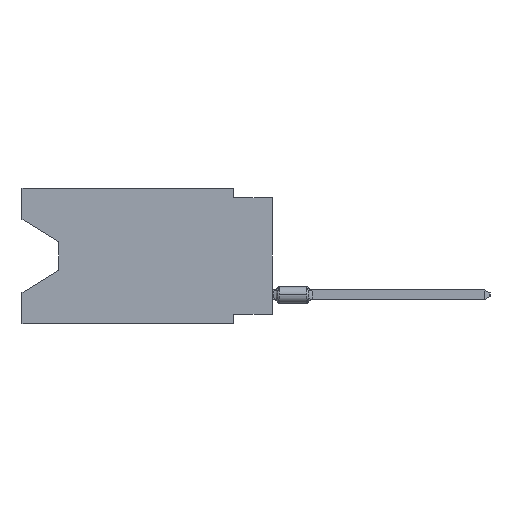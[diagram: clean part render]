
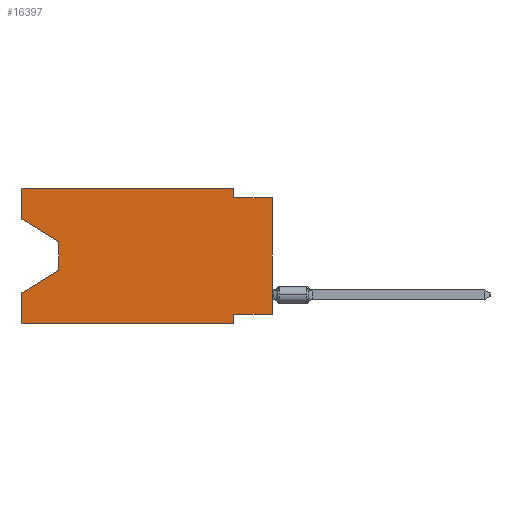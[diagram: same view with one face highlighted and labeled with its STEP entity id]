
A CAD part, left-side view. The second image highlights one B-rep face of the part: STEP entity #16397.
In plain terms, the highlighted planar face has unit normal (-1, 0, 0).
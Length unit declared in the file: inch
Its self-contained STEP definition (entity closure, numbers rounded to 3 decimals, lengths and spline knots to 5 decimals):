
#1196 = DIRECTION ( 'NONE',  ( 0., 0., -1. ) ) ;
#1961 = EDGE_CURVE ( 'NONE', #27140, #8039, #2469, .T. ) ;
#2184 = VECTOR ( 'NONE', #6660, 39.37008 ) ;
#2469 = LINE ( 'NONE', #33459, #2823 ) ;
#2578 = DIRECTION ( 'NONE',  ( 0., 1., 0. ) ) ;
#2591 = CARTESIAN_POINT ( 'NONE',  ( 0., 0., -0.025 ) ) ;
#2623 = VECTOR ( 'NONE', #19861, 39.37008 ) ;
#2651 = ORIENTED_EDGE ( 'NONE', *, *, #20667, .T. ) ;
#2823 = VECTOR ( 'NONE', #5797, 39.37008 ) ;
#2861 = CARTESIAN_POINT ( 'NONE',  ( 0., 0.645, -0.35 ) ) ;
#3472 = CARTESIAN_POINT ( 'NONE',  ( 0., 0.55, -0.138 ) ) ;
#3521 = FACE_OUTER_BOUND ( 'NONE', #13772, .T. ) ;
#3832 = VERTEX_POINT ( 'NONE', #13903 ) ;
#3996 = ORIENTED_EDGE ( 'NONE', *, *, #23947, .F. ) ;
#4354 = VECTOR ( 'NONE', #19300, 39.37008 ) ;
#4499 = ORIENTED_EDGE ( 'NONE', *, *, #34198, .F. ) ;
#4878 = CARTESIAN_POINT ( 'NONE',  ( 0., 0.1, -0.325 ) ) ;
#5626 = ORIENTED_EDGE ( 'NONE', *, *, #24805, .T. ) ;
#5797 = DIRECTION ( 'NONE',  ( 0., 0., -1. ) ) ;
#5922 = CARTESIAN_POINT ( 'NONE',  ( 0., 0., 0. ) ) ;
#6173 = VERTEX_POINT ( 'NONE', #33306 ) ;
#6267 = VECTOR ( 'NONE', #35871, 39.37008 ) ;
#6556 = LINE ( 'NONE', #35153, #23487 ) ;
#6660 = DIRECTION ( 'NONE',  ( 0., 0., 1. ) ) ;
#6826 = EDGE_CURVE ( 'NONE', #9993, #15553, #34733, .T. ) ;
#7477 = LINE ( 'NONE', #18599, #6267 ) ;
#7908 = VECTOR ( 'NONE', #35637, 39.37008 ) ;
#8039 = VERTEX_POINT ( 'NONE', #25841 ) ;
#8499 = VECTOR ( 'NONE', #20613, 39.37008 ) ;
#9249 = VECTOR ( 'NONE', #2578, 39.37008 ) ;
#9289 = CARTESIAN_POINT ( 'NONE',  ( 0., 0.645, -0.08025 ) ) ;
#9309 = CARTESIAN_POINT ( 'NONE',  ( 0., 0., -0.025 ) ) ;
#9993 = VERTEX_POINT ( 'NONE', #21001 ) ;
#10568 = LINE ( 'NONE', #21866, #9249 ) ;
#10774 = CARTESIAN_POINT ( 'NONE',  ( 0., 0.645, 0. ) ) ;
#11187 = CARTESIAN_POINT ( 'NONE',  ( 0., 0.645, 0. ) ) ;
#11230 = DIRECTION ( 'NONE',  ( 0., -1., 0. ) ) ;
#11483 = CARTESIAN_POINT ( 'NONE',  ( 0., 0.645, 0. ) ) ;
#11693 = LINE ( 'NONE', #5922, #2623 ) ;
#12108 = EDGE_CURVE ( 'NONE', #33891, #9993, #7477, .T. ) ;
#12478 = EDGE_CURVE ( 'NONE', #28053, #20591, #25641, .T. ) ;
#12960 = CARTESIAN_POINT ( 'NONE',  ( 0., 0.1, -0.35 ) ) ;
#13772 = EDGE_LOOP ( 'NONE', ( #15300, #21394, #2651, #24624, #5626, #32148, #3996, #18619, #17674, #19186, #4499, #22577 ) ) ;
#13903 = CARTESIAN_POINT ( 'NONE',  ( 0., 0.645, -0.35 ) ) ;
#14353 = LINE ( 'NONE', #2861, #31803 ) ;
#14556 = AXIS2_PLACEMENT_3D ( 'NONE', #31385, #17991, #29315 ) ;
#15300 = ORIENTED_EDGE ( 'NONE', *, *, #24706, .T. ) ;
#15553 = VERTEX_POINT ( 'NONE', #2591 ) ;
#15781 = CARTESIAN_POINT ( 'NONE',  ( 0., 0.55, -0.212 ) ) ;
#15980 = LINE ( 'NONE', #11187, #30486 ) ;
#16159 = DIRECTION ( 'NONE',  ( 0., -1., 0. ) ) ;
#16397 = ADVANCED_FACE ( 'NONE', ( #3521 ), #29113, .F. ) ;
#16633 = CARTESIAN_POINT ( 'NONE',  ( 0., 0., -0.325 ) ) ;
#17674 = ORIENTED_EDGE ( 'NONE', *, *, #6826, .F. ) ;
#17991 = DIRECTION ( 'NONE',  ( 1., 0., 0. ) ) ;
#18599 = CARTESIAN_POINT ( 'NONE',  ( 0., 0.1, 0. ) ) ;
#18619 = ORIENTED_EDGE ( 'NONE', *, *, #20773, .T. ) ;
#18996 = LINE ( 'NONE', #21960, #19373 ) ;
#19186 = ORIENTED_EDGE ( 'NONE', *, *, #12108, .F. ) ;
#19300 = DIRECTION ( 'NONE',  ( 0., 0., 1. ) ) ;
#19373 = VECTOR ( 'NONE', #22351, 39.37008 ) ;
#19861 = DIRECTION ( 'NONE',  ( 0., 0., 1. ) ) ;
#20225 = VERTEX_POINT ( 'NONE', #12960 ) ;
#20239 = CARTESIAN_POINT ( 'NONE',  ( 0., 0.645, 0. ) ) ;
#20591 = VERTEX_POINT ( 'NONE', #10774 ) ;
#20613 = DIRECTION ( 'NONE',  ( 0., -1., 0. ) ) ;
#20667 = EDGE_CURVE ( 'NONE', #8039, #6173, #32652, .T. ) ;
#20773 = EDGE_CURVE ( 'NONE', #23148, #15553, #11693, .T. ) ;
#21001 = CARTESIAN_POINT ( 'NONE',  ( 0., 0.1, -0.025 ) ) ;
#21394 = ORIENTED_EDGE ( 'NONE', *, *, #1961, .T. ) ;
#21866 = CARTESIAN_POINT ( 'NONE',  ( 0., 0., -0.325 ) ) ;
#21960 = CARTESIAN_POINT ( 'NONE',  ( 0., 0.645, -0.08025 ) ) ;
#22351 = DIRECTION ( 'NONE',  ( 0., -0.855, -0.519 ) ) ;
#22577 = ORIENTED_EDGE ( 'NONE', *, *, #12478, .F. ) ;
#22797 = LINE ( 'NONE', #11483, #4354 ) ;
#23148 = VERTEX_POINT ( 'NONE', #16633 ) ;
#23487 = VECTOR ( 'NONE', #1196, 39.37008 ) ;
#23947 = EDGE_CURVE ( 'NONE', #23148, #26241, #10568, .T. ) ;
#24564 = EDGE_CURVE ( 'NONE', #26241, #20225, #6556, .T. ) ;
#24587 = CARTESIAN_POINT ( 'NONE',  ( 0., 0.1, 0. ) ) ;
#24624 = ORIENTED_EDGE ( 'NONE', *, *, #33042, .F. ) ;
#24706 = EDGE_CURVE ( 'NONE', #28053, #27140, #18996, .T. ) ;
#24805 = EDGE_CURVE ( 'NONE', #3832, #20225, #14353, .T. ) ;
#25641 = LINE ( 'NONE', #20239, #2184 ) ;
#25841 = CARTESIAN_POINT ( 'NONE',  ( 0., 0.55, -0.212 ) ) ;
#26241 = VERTEX_POINT ( 'NONE', #4878 ) ;
#27140 = VERTEX_POINT ( 'NONE', #3472 ) ;
#28053 = VERTEX_POINT ( 'NONE', #9289 ) ;
#29113 = PLANE ( 'NONE',  #14556 ) ;
#29315 = DIRECTION ( 'NONE',  ( 0., 0., -1. ) ) ;
#30486 = VECTOR ( 'NONE', #16159, 39.37008 ) ;
#31385 = CARTESIAN_POINT ( 'NONE',  ( 0., 0.645, 0. ) ) ;
#31803 = VECTOR ( 'NONE', #11230, 39.37008 ) ;
#32148 = ORIENTED_EDGE ( 'NONE', *, *, #24564, .F. ) ;
#32652 = LINE ( 'NONE', #15781, #7908 ) ;
#33042 = EDGE_CURVE ( 'NONE', #3832, #6173, #22797, .T. ) ;
#33306 = CARTESIAN_POINT ( 'NONE',  ( 0., 0.645, -0.26975 ) ) ;
#33459 = CARTESIAN_POINT ( 'NONE',  ( 0., 0.55, -0.138 ) ) ;
#33891 = VERTEX_POINT ( 'NONE', #24587 ) ;
#34198 = EDGE_CURVE ( 'NONE', #20591, #33891, #15980, .T. ) ;
#34733 = LINE ( 'NONE', #9309, #8499 ) ;
#35153 = CARTESIAN_POINT ( 'NONE',  ( 0., 0.1, -0.35 ) ) ;
#35637 = DIRECTION ( 'NONE',  ( 0., 0.855, -0.519 ) ) ;
#35871 = DIRECTION ( 'NONE',  ( 0., 0., -1. ) ) ;
